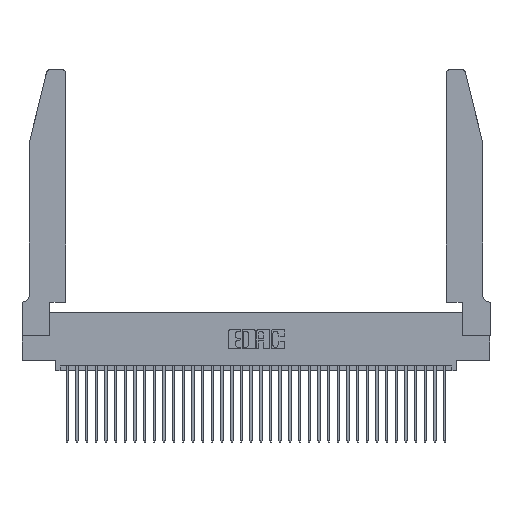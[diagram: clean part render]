
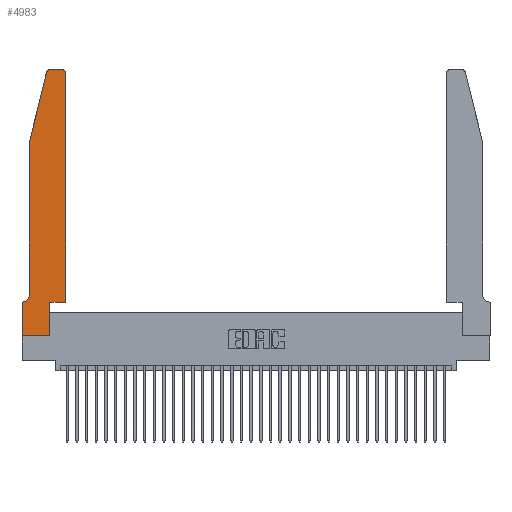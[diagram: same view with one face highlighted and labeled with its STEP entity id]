
A CAD part, top view. The second image highlights one B-rep face of the part: STEP entity #4983.
In plain terms, the highlighted planar face has unit normal (0, 0, 1).
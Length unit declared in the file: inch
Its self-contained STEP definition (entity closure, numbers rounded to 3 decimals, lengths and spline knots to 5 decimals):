
#369 = CIRCLE ( 'NONE', #26322, 0.03 ) ;
#1698 = FACE_OUTER_BOUND ( 'NONE', #25820, .T. ) ;
#1717 = DIRECTION ( 'NONE',  ( 0., 0., 1. ) ) ;
#1727 = VECTOR ( 'NONE', #29928, 39.37008 ) ;
#2017 = EDGE_CURVE ( 'NONE', #31505, #9287, #12203, .T. ) ;
#3119 = DIRECTION ( 'NONE',  ( 0., 0., 1. ) ) ;
#3192 = LINE ( 'NONE', #26743, #33215 ) ;
#3405 = DIRECTION ( 'NONE',  ( 0., -1., 0. ) ) ;
#3579 = EDGE_CURVE ( 'NONE', #5114, #4603, #24482, .T. ) ;
#4603 = VERTEX_POINT ( 'NONE', #28387 ) ;
#4983 = ADVANCED_FACE ( 'NONE', ( #1698 ), #29940, .T. ) ;
#5071 = EDGE_CURVE ( 'NONE', #15658, #22210, #6645, .T. ) ;
#5114 = VERTEX_POINT ( 'NONE', #30542 ) ;
#5459 = EDGE_CURVE ( 'NONE', #35804, #25249, #17337, .T. ) ;
#6458 = CARTESIAN_POINT ( 'NONE',  ( 0.284, 2.72, 0.37 ) ) ;
#6645 = LINE ( 'NONE', #30419, #36555 ) ;
#6739 = VECTOR ( 'NONE', #29425, 39.37008 ) ;
#6836 = CARTESIAN_POINT ( 'NONE',  ( 0., 0., 0.37 ) ) ;
#7669 = EDGE_CURVE ( 'NONE', #8238, #32141, #3192, .T. ) ;
#8203 = CARTESIAN_POINT ( 'NONE',  ( 0.0755, 0.42, 0.37 ) ) ;
#8238 = VERTEX_POINT ( 'NONE', #28985 ) ;
#8382 = CARTESIAN_POINT ( 'NONE',  ( 0.0755, 0.35, 0.37 ) ) ;
#8711 = EDGE_CURVE ( 'NONE', #10632, #15658, #369, .T. ) ;
#8931 = EDGE_CURVE ( 'NONE', #34760, #8238, #22632, .T. ) ;
#9287 = VERTEX_POINT ( 'NONE', #21961 ) ;
#9318 = DIRECTION ( 'NONE',  ( 1., 0., 0. ) ) ;
#9337 = DIRECTION ( 'NONE',  ( 0., 0., -1. ) ) ;
#9785 = DIRECTION ( 'NONE',  ( 0., -1., 0. ) ) ;
#9790 = VECTOR ( 'NONE', #31973, 39.37008 ) ;
#10562 = ORIENTED_EDGE ( 'NONE', *, *, #5459, .T. ) ;
#10632 = VERTEX_POINT ( 'NONE', #16444 ) ;
#11028 = ORIENTED_EDGE ( 'NONE', *, *, #31948, .T. ) ;
#11569 = CARTESIAN_POINT ( 'NONE',  ( 0.25487, 2.72718, 0.37 ) ) ;
#11931 = AXIS2_PLACEMENT_3D ( 'NONE', #26291, #9337, #29063 ) ;
#12179 = CARTESIAN_POINT ( 'NONE',  ( 0.4505, 0.35, 0.37 ) ) ;
#12203 = LINE ( 'NONE', #8382, #27226 ) ;
#12566 = DIRECTION ( 'NONE',  ( -0.239, -0.971, 0. ) ) ;
#12635 = ORIENTED_EDGE ( 'NONE', *, *, #8931, .T. ) ;
#13585 = DIRECTION ( 'NONE',  ( -1., 0., 0. ) ) ;
#15118 = VECTOR ( 'NONE', #12566, 39.37008 ) ;
#15505 = CARTESIAN_POINT ( 'NONE',  ( 0.4505, 0.35, 0.37 ) ) ;
#15658 = VERTEX_POINT ( 'NONE', #26337 ) ;
#16331 = EDGE_CURVE ( 'NONE', #32141, #31505, #27092, .T. ) ;
#16444 = CARTESIAN_POINT ( 'NONE',  ( 0.4505, 2.72, 0.37 ) ) ;
#17337 = LINE ( 'NONE', #12179, #9790 ) ;
#18178 = ORIENTED_EDGE ( 'NONE', *, *, #2017, .T. ) ;
#18491 = EDGE_CURVE ( 'NONE', #25249, #10632, #30884, .T. ) ;
#18608 = ORIENTED_EDGE ( 'NONE', *, *, #27755, .T. ) ;
#18644 = ORIENTED_EDGE ( 'NONE', *, *, #16331, .T. ) ;
#18776 = CARTESIAN_POINT ( 'NONE',  ( 0.2865, 0.35, 0.37 ) ) ;
#18787 = CARTESIAN_POINT ( 'NONE',  ( 0., 0.35, 0.37 ) ) ;
#18920 = ORIENTED_EDGE ( 'NONE', *, *, #8711, .T. ) ;
#20066 = CARTESIAN_POINT ( 'NONE',  ( 0.4505, 0.35, 0.37 ) ) ;
#20139 = CARTESIAN_POINT ( 'NONE',  ( 0.4205, 2.72, 0.37 ) ) ;
#20250 = LINE ( 'NONE', #34480, #34237 ) ;
#20870 = CIRCLE ( 'NONE', #24642, 0.03 ) ;
#21608 = DIRECTION ( 'NONE',  ( 1., 0., 0. ) ) ;
#21961 = CARTESIAN_POINT ( 'NONE',  ( 0., 0.35, 0.37 ) ) ;
#22210 = VERTEX_POINT ( 'NONE', #31977 ) ;
#22632 = LINE ( 'NONE', #26669, #15118 ) ;
#22966 = DIRECTION ( 'NONE',  ( 1., 0., 0. ) ) ;
#24342 = VECTOR ( 'NONE', #32324, 39.37008 ) ;
#24482 = LINE ( 'NONE', #6836, #6739 ) ;
#24597 = AXIS2_PLACEMENT_3D ( 'NONE', #18787, #1717, #21608 ) ;
#24642 = AXIS2_PLACEMENT_3D ( 'NONE', #6458, #26271, #9318 ) ;
#24990 = CARTESIAN_POINT ( 'NONE',  ( 0.0055, 0.35, 0.37 ) ) ;
#25249 = VERTEX_POINT ( 'NONE', #20066 ) ;
#25820 = EDGE_LOOP ( 'NONE', ( #32909, #33323, #12635, #28473, #18644, #18178, #18608, #32175, #11028, #10562, #26885, #18920 ) ) ;
#25961 = CARTESIAN_POINT ( 'NONE',  ( 0.2865, 0.35, 0.37 ) ) ;
#26271 = DIRECTION ( 'NONE',  ( 0., 0., 1. ) ) ;
#26291 = CARTESIAN_POINT ( 'NONE',  ( 0.0055, 0.42, 0.37 ) ) ;
#26322 = AXIS2_PLACEMENT_3D ( 'NONE', #20139, #3119, #22966 ) ;
#26337 = CARTESIAN_POINT ( 'NONE',  ( 0.4205, 2.75, 0.37 ) ) ;
#26669 = CARTESIAN_POINT ( 'NONE',  ( 0.0755, 2., 0.37 ) ) ;
#26743 = CARTESIAN_POINT ( 'NONE',  ( 0.0755, 2., 0.37 ) ) ;
#26885 = ORIENTED_EDGE ( 'NONE', *, *, #18491, .T. ) ;
#27092 = CIRCLE ( 'NONE', #11931, 0.07 ) ;
#27226 = VECTOR ( 'NONE', #30945, 39.37008 ) ;
#27755 = EDGE_CURVE ( 'NONE', #9287, #5114, #20250, .T. ) ;
#28387 = CARTESIAN_POINT ( 'NONE',  ( 0.2865, 0., 0.37 ) ) ;
#28473 = ORIENTED_EDGE ( 'NONE', *, *, #7669, .T. ) ;
#28985 = CARTESIAN_POINT ( 'NONE',  ( 0.0755, 2., 0.37 ) ) ;
#29063 = DIRECTION ( 'NONE',  ( -1., 0., 0. ) ) ;
#29425 = DIRECTION ( 'NONE',  ( 1., 0., 0. ) ) ;
#29928 = DIRECTION ( 'NONE',  ( 0., 1., 0. ) ) ;
#29940 = PLANE ( 'NONE',  #24597 ) ;
#30419 = CARTESIAN_POINT ( 'NONE',  ( 0.2605, 2.75, 0.37 ) ) ;
#30542 = CARTESIAN_POINT ( 'NONE',  ( 0., 0., 0.37 ) ) ;
#30884 = LINE ( 'NONE', #15505, #24342 ) ;
#30945 = DIRECTION ( 'NONE',  ( -1., 0., 0. ) ) ;
#30948 = LINE ( 'NONE', #18776, #1727 ) ;
#31505 = VERTEX_POINT ( 'NONE', #24990 ) ;
#31948 = EDGE_CURVE ( 'NONE', #4603, #35804, #30948, .T. ) ;
#31973 = DIRECTION ( 'NONE',  ( 1., 0., 0. ) ) ;
#31977 = CARTESIAN_POINT ( 'NONE',  ( 0.284, 2.75, 0.37 ) ) ;
#32141 = VERTEX_POINT ( 'NONE', #8203 ) ;
#32175 = ORIENTED_EDGE ( 'NONE', *, *, #3579, .T. ) ;
#32324 = DIRECTION ( 'NONE',  ( 0., 1., 0. ) ) ;
#32909 = ORIENTED_EDGE ( 'NONE', *, *, #5071, .T. ) ;
#33215 = VECTOR ( 'NONE', #9785, 39.37008 ) ;
#33239 = EDGE_CURVE ( 'NONE', #22210, #34760, #20870, .T. ) ;
#33323 = ORIENTED_EDGE ( 'NONE', *, *, #33239, .T. ) ;
#34237 = VECTOR ( 'NONE', #3405, 39.37008 ) ;
#34480 = CARTESIAN_POINT ( 'NONE',  ( 0., 0., 0.37 ) ) ;
#34760 = VERTEX_POINT ( 'NONE', #11569 ) ;
#35804 = VERTEX_POINT ( 'NONE', #25961 ) ;
#36555 = VECTOR ( 'NONE', #13585, 39.37008 ) ;
